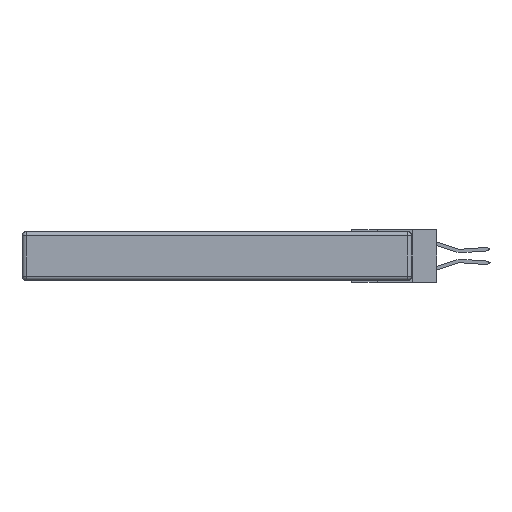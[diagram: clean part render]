
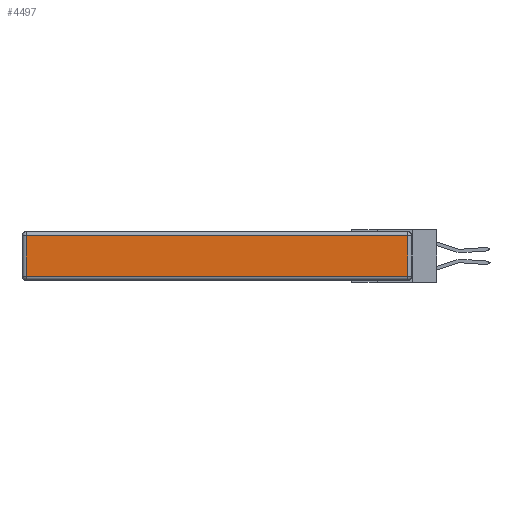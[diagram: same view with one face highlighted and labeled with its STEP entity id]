
A CAD part, left-side view. The second image highlights one B-rep face of the part: STEP entity #4497.
In plain terms, the highlighted planar face has unit normal (-1, 0, 0).
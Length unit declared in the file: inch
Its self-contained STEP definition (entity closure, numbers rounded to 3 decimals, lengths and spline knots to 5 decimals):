
#782 = VERTEX_POINT ( 'NONE', #4409 ) ;
#1458 = DIRECTION ( 'NONE',  ( 0., 0., 1. ) ) ;
#1746 = CARTESIAN_POINT ( 'NONE',  ( 0., 0.03, -0.313 ) ) ;
#2133 = VECTOR ( 'NONE', #6589, 39.37008 ) ;
#2191 = CARTESIAN_POINT ( 'NONE',  ( 0., 0., -0.313 ) ) ;
#2403 = CARTESIAN_POINT ( 'NONE',  ( 0., 2.72, -0.313 ) ) ;
#2481 = VECTOR ( 'NONE', #15960, 39.37008 ) ;
#2503 = AXIS2_PLACEMENT_3D ( 'NONE', #4140, #8547, #4464 ) ;
#2601 = EDGE_CURVE ( 'NONE', #10542, #9747, #7579, .T. ) ;
#3485 = CARTESIAN_POINT ( 'NONE',  ( 0., 2.72, -0.343 ) ) ;
#4140 = CARTESIAN_POINT ( 'NONE',  ( 0., 0., -0.343 ) ) ;
#4409 = CARTESIAN_POINT ( 'NONE',  ( 0., 0.03, -0.03 ) ) ;
#4464 = DIRECTION ( 'NONE',  ( 0., 0., 1. ) ) ;
#4497 = ADVANCED_FACE ( 'NONE', ( #9815 ), #17131, .T. ) ;
#4852 = VERTEX_POINT ( 'NONE', #1746 ) ;
#5631 = CARTESIAN_POINT ( 'NONE',  ( 0., 0.03, -0.343 ) ) ;
#5841 = CARTESIAN_POINT ( 'NONE',  ( 0., 2.75, -0.03 ) ) ;
#6589 = DIRECTION ( 'NONE',  ( 0., 0., -1. ) ) ;
#7261 = VECTOR ( 'NONE', #1458, 39.37008 ) ;
#7579 = LINE ( 'NONE', #3485, #2133 ) ;
#7645 = ORIENTED_EDGE ( 'NONE', *, *, #2601, .T. ) ;
#7739 = LINE ( 'NONE', #5631, #7261 ) ;
#8547 = DIRECTION ( 'NONE',  ( -1., 0., 0. ) ) ;
#9747 = VERTEX_POINT ( 'NONE', #2403 ) ;
#9815 = FACE_OUTER_BOUND ( 'NONE', #11942, .T. ) ;
#9977 = EDGE_CURVE ( 'NONE', #4852, #782, #7739, .T. ) ;
#10520 = ORIENTED_EDGE ( 'NONE', *, *, #17592, .T. ) ;
#10542 = VERTEX_POINT ( 'NONE', #18713 ) ;
#11942 = EDGE_LOOP ( 'NONE', ( #16497, #15387, #10520, #7645 ) ) ;
#12608 = LINE ( 'NONE', #2191, #13521 ) ;
#13521 = VECTOR ( 'NONE', #15669, 39.37008 ) ;
#14390 = EDGE_CURVE ( 'NONE', #9747, #4852, #12608, .T. ) ;
#15387 = ORIENTED_EDGE ( 'NONE', *, *, #9977, .T. ) ;
#15669 = DIRECTION ( 'NONE',  ( 0., -1., 0. ) ) ;
#15960 = DIRECTION ( 'NONE',  ( 0., 1., 0. ) ) ;
#16497 = ORIENTED_EDGE ( 'NONE', *, *, #14390, .T. ) ;
#17131 = PLANE ( 'NONE',  #2503 ) ;
#17592 = EDGE_CURVE ( 'NONE', #782, #10542, #17934, .T. ) ;
#17934 = LINE ( 'NONE', #5841, #2481 ) ;
#18713 = CARTESIAN_POINT ( 'NONE',  ( 0., 2.72, -0.03 ) ) ;
